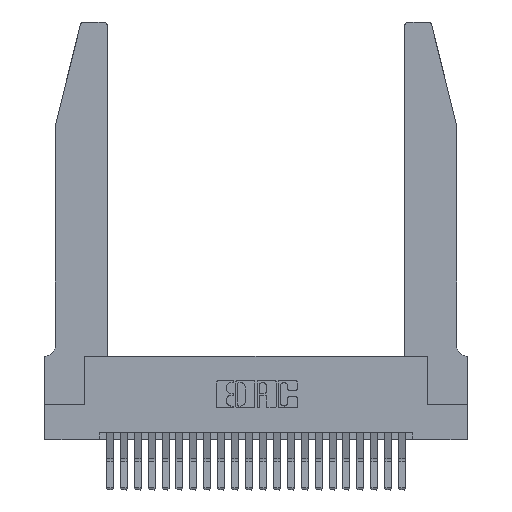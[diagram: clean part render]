
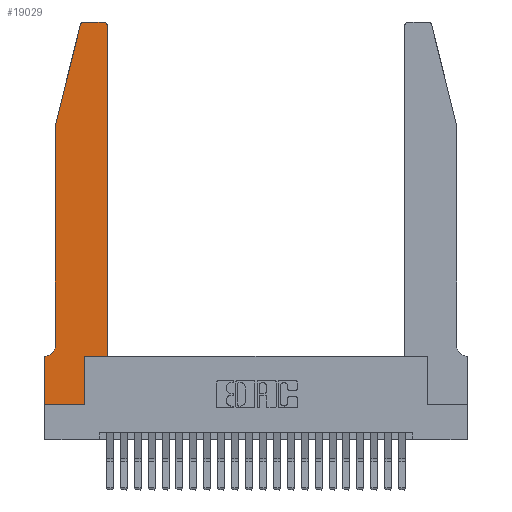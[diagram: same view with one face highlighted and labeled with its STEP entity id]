
A CAD part, top view. The second image highlights one B-rep face of the part: STEP entity #19029.
In plain terms, the highlighted planar face has unit normal (0, 0, 1).
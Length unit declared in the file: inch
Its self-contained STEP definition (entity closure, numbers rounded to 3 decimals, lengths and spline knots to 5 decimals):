
#545 = CARTESIAN_POINT ( 'NONE',  ( 0.2605, 2.75, 0.37 ) ) ;
#960 = ORIENTED_EDGE ( 'NONE', *, *, #6667, .T. ) ;
#1066 = ORIENTED_EDGE ( 'NONE', *, *, #14751, .T. ) ;
#1122 = EDGE_CURVE ( 'NONE', #12180, #9307, #15405, .T. ) ;
#1144 = CIRCLE ( 'NONE', #19045, 0.03 ) ;
#1636 = DIRECTION ( 'NONE',  ( 0., 0., 1. ) ) ;
#1845 = ORIENTED_EDGE ( 'NONE', *, *, #8905, .T. ) ;
#1863 = DIRECTION ( 'NONE',  ( 0., 1., 0. ) ) ;
#2542 = DIRECTION ( 'NONE',  ( -1., 0., 0. ) ) ;
#3004 = LINE ( 'NONE', #11562, #17216 ) ;
#3059 = VECTOR ( 'NONE', #23011, 39.37008 ) ;
#3287 = VERTEX_POINT ( 'NONE', #24787 ) ;
#3797 = CARTESIAN_POINT ( 'NONE',  ( 0.4205, 2.75, 0.37 ) ) ;
#3813 = VERTEX_POINT ( 'NONE', #10995 ) ;
#3950 = LINE ( 'NONE', #10954, #19923 ) ;
#4248 = VECTOR ( 'NONE', #1863, 39.37008 ) ;
#5147 = EDGE_CURVE ( 'NONE', #3813, #16741, #3950, .T. ) ;
#5880 = CARTESIAN_POINT ( 'NONE',  ( 0.0055, 0.42, 0.37 ) ) ;
#5884 = EDGE_CURVE ( 'NONE', #6766, #3813, #9164, .T. ) ;
#6195 = VERTEX_POINT ( 'NONE', #17894 ) ;
#6244 = DIRECTION ( 'NONE',  ( 1., 0., 0. ) ) ;
#6667 = EDGE_CURVE ( 'NONE', #22230, #23611, #3004, .T. ) ;
#6766 = VERTEX_POINT ( 'NONE', #11820 ) ;
#7801 = CARTESIAN_POINT ( 'NONE',  ( 0.2865, 0.35, 0.37 ) ) ;
#7859 = DIRECTION ( 'NONE',  ( -1., 0., 0. ) ) ;
#8069 = CARTESIAN_POINT ( 'NONE',  ( 0.4205, 2.72, 0.37 ) ) ;
#8873 = LINE ( 'NONE', #7801, #3059 ) ;
#8905 = EDGE_CURVE ( 'NONE', #16741, #22003, #13853, .T. ) ;
#9149 = CARTESIAN_POINT ( 'NONE',  ( 0.2865, 0.35, 0.37 ) ) ;
#9164 = LINE ( 'NONE', #22708, #18724 ) ;
#9307 = VERTEX_POINT ( 'NONE', #11297 ) ;
#10038 = DIRECTION ( 'NONE',  ( 1., 0., 0. ) ) ;
#10074 = LINE ( 'NONE', #11580, #4248 ) ;
#10695 = AXIS2_PLACEMENT_3D ( 'NONE', #22870, #11597, #24720 ) ;
#10875 = EDGE_LOOP ( 'NONE', ( #22165, #11050, #18845, #960, #17055, #23015, #14252, #1845, #16712, #19677, #15909, #1066 ) ) ;
#10954 = CARTESIAN_POINT ( 'NONE',  ( 0., 0., 0.37 ) ) ;
#10995 = CARTESIAN_POINT ( 'NONE',  ( 0., 0.35, 0.37 ) ) ;
#11050 = ORIENTED_EDGE ( 'NONE', *, *, #21958, .T. ) ;
#11297 = CARTESIAN_POINT ( 'NONE',  ( 0.4505, 0.35, 0.37 ) ) ;
#11401 = CIRCLE ( 'NONE', #10695, 0.03 ) ;
#11562 = CARTESIAN_POINT ( 'NONE',  ( 0.0755, 2., 0.37 ) ) ;
#11580 = CARTESIAN_POINT ( 'NONE',  ( 0.4505, 0.35, 0.37 ) ) ;
#11597 = DIRECTION ( 'NONE',  ( 0., 0., 1. ) ) ;
#11820 = CARTESIAN_POINT ( 'NONE',  ( 0.0055, 0.35, 0.37 ) ) ;
#12180 = VERTEX_POINT ( 'NONE', #9149 ) ;
#12387 = CIRCLE ( 'NONE', #15305, 0.07 ) ;
#12498 = EDGE_CURVE ( 'NONE', #3287, #22230, #18977, .T. ) ;
#12739 = EDGE_CURVE ( 'NONE', #9307, #22004, #10074, .T. ) ;
#13280 = PLANE ( 'NONE',  #13729 ) ;
#13729 = AXIS2_PLACEMENT_3D ( 'NONE', #18898, #1636, #15211 ) ;
#13853 = LINE ( 'NONE', #19708, #18859 ) ;
#13978 = VECTOR ( 'NONE', #19588, 39.37008 ) ;
#14252 = ORIENTED_EDGE ( 'NONE', *, *, #5147, .T. ) ;
#14625 = VERTEX_POINT ( 'NONE', #3797 ) ;
#14751 = EDGE_CURVE ( 'NONE', #22004, #14625, #1144, .T. ) ;
#14781 = CARTESIAN_POINT ( 'NONE',  ( 0.4505, 0.35, 0.37 ) ) ;
#15211 = DIRECTION ( 'NONE',  ( 1., 0., 0. ) ) ;
#15305 = AXIS2_PLACEMENT_3D ( 'NONE', #5880, #19350, #7859 ) ;
#15365 = LINE ( 'NONE', #545, #24680 ) ;
#15405 = LINE ( 'NONE', #14781, #19836 ) ;
#15806 = CARTESIAN_POINT ( 'NONE',  ( 0.0755, 2., 0.37 ) ) ;
#15909 = ORIENTED_EDGE ( 'NONE', *, *, #12739, .T. ) ;
#16185 = EDGE_CURVE ( 'NONE', #14625, #6195, #15365, .T. ) ;
#16320 = CARTESIAN_POINT ( 'NONE',  ( 0., 0., 0.37 ) ) ;
#16712 = ORIENTED_EDGE ( 'NONE', *, *, #19796, .T. ) ;
#16741 = VERTEX_POINT ( 'NONE', #16320 ) ;
#17055 = ORIENTED_EDGE ( 'NONE', *, *, #17098, .T. ) ;
#17098 = EDGE_CURVE ( 'NONE', #23611, #6766, #12387, .T. ) ;
#17216 = VECTOR ( 'NONE', #24689, 39.37008 ) ;
#17894 = CARTESIAN_POINT ( 'NONE',  ( 0.284, 2.75, 0.37 ) ) ;
#18055 = CARTESIAN_POINT ( 'NONE',  ( 0.0755, 2., 0.37 ) ) ;
#18724 = VECTOR ( 'NONE', #24561, 39.37008 ) ;
#18845 = ORIENTED_EDGE ( 'NONE', *, *, #12498, .T. ) ;
#18859 = VECTOR ( 'NONE', #6244, 39.37008 ) ;
#18898 = CARTESIAN_POINT ( 'NONE',  ( 0., 0.35, 0.37 ) ) ;
#18977 = LINE ( 'NONE', #15806, #13978 ) ;
#19029 = ADVANCED_FACE ( 'NONE', ( #19388 ), #13280, .T. ) ;
#19045 = AXIS2_PLACEMENT_3D ( 'NONE', #8069, #21425, #10038 ) ;
#19312 = CARTESIAN_POINT ( 'NONE',  ( 0.2865, 0., 0.37 ) ) ;
#19350 = DIRECTION ( 'NONE',  ( 0., 0., -1. ) ) ;
#19388 = FACE_OUTER_BOUND ( 'NONE', #10875, .T. ) ;
#19588 = DIRECTION ( 'NONE',  ( -0.239, -0.971, 0. ) ) ;
#19677 = ORIENTED_EDGE ( 'NONE', *, *, #1122, .T. ) ;
#19708 = CARTESIAN_POINT ( 'NONE',  ( 0., 0., 0.37 ) ) ;
#19796 = EDGE_CURVE ( 'NONE', #22003, #12180, #8873, .T. ) ;
#19836 = VECTOR ( 'NONE', #22321, 39.37008 ) ;
#19923 = VECTOR ( 'NONE', #24108, 39.37008 ) ;
#21116 = CARTESIAN_POINT ( 'NONE',  ( 0.4505, 2.72, 0.37 ) ) ;
#21282 = CARTESIAN_POINT ( 'NONE',  ( 0.0755, 0.42, 0.37 ) ) ;
#21425 = DIRECTION ( 'NONE',  ( 0., 0., 1. ) ) ;
#21958 = EDGE_CURVE ( 'NONE', #6195, #3287, #11401, .T. ) ;
#22003 = VERTEX_POINT ( 'NONE', #19312 ) ;
#22004 = VERTEX_POINT ( 'NONE', #21116 ) ;
#22165 = ORIENTED_EDGE ( 'NONE', *, *, #16185, .T. ) ;
#22230 = VERTEX_POINT ( 'NONE', #18055 ) ;
#22321 = DIRECTION ( 'NONE',  ( 1., 0., 0. ) ) ;
#22708 = CARTESIAN_POINT ( 'NONE',  ( 0.0755, 0.35, 0.37 ) ) ;
#22870 = CARTESIAN_POINT ( 'NONE',  ( 0.284, 2.72, 0.37 ) ) ;
#23011 = DIRECTION ( 'NONE',  ( 0., 1., 0. ) ) ;
#23015 = ORIENTED_EDGE ( 'NONE', *, *, #5884, .T. ) ;
#23611 = VERTEX_POINT ( 'NONE', #21282 ) ;
#24108 = DIRECTION ( 'NONE',  ( 0., -1., 0. ) ) ;
#24561 = DIRECTION ( 'NONE',  ( -1., 0., 0. ) ) ;
#24680 = VECTOR ( 'NONE', #2542, 39.37008 ) ;
#24689 = DIRECTION ( 'NONE',  ( 0., -1., 0. ) ) ;
#24720 = DIRECTION ( 'NONE',  ( 1., 0., 0. ) ) ;
#24787 = CARTESIAN_POINT ( 'NONE',  ( 0.25487, 2.72718, 0.37 ) ) ;
